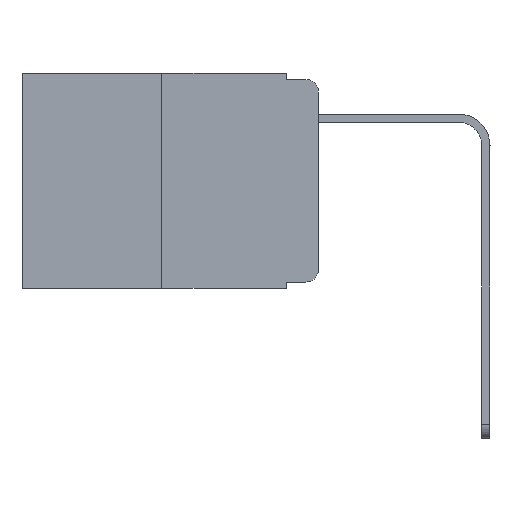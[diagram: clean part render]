
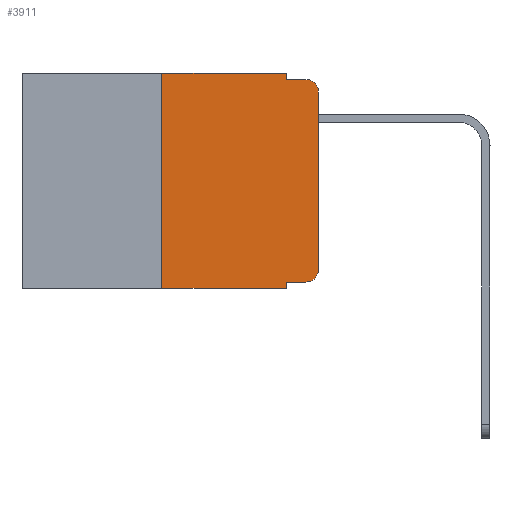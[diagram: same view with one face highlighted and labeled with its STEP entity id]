
A CAD part, left-side view. The second image highlights one B-rep face of the part: STEP entity #3911.
In plain terms, the highlighted planar face has unit normal (-1, 0, 0).
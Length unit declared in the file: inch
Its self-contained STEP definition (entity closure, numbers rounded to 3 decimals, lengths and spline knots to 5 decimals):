
#37 = DIRECTION ( 'NONE',  ( 0., -1., 0. ) ) ;
#202 = LINE ( 'NONE', #6691, #6022 ) ;
#251 = EDGE_CURVE ( 'NONE', #5769, #3876, #7273, .T. ) ;
#283 = DIRECTION ( 'NONE',  ( 0., 0., 1. ) ) ;
#401 = CARTESIAN_POINT ( 'NONE',  ( 0., 0.02, -0.03 ) ) ;
#458 = DIRECTION ( 'NONE',  ( -1., 0., 0. ) ) ;
#551 = CIRCLE ( 'NONE', #3579, 0.02 ) ;
#652 = EDGE_CURVE ( 'NONE', #7943, #8433, #551, .T. ) ;
#853 = VERTEX_POINT ( 'NONE', #8918 ) ;
#938 = CARTESIAN_POINT ( 'NONE',  ( 0., 0.473, -0.343 ) ) ;
#1070 = AXIS2_PLACEMENT_3D ( 'NONE', #401, #7732, #2834 ) ;
#1266 = EDGE_LOOP ( 'NONE', ( #7208, #2586, #8541, #6045, #2833, #6944, #1284, #6543, #9168, #8467 ) ) ;
#1284 = ORIENTED_EDGE ( 'NONE', *, *, #10166, .T. ) ;
#1497 = CARTESIAN_POINT ( 'NONE',  ( 0., 0., -0.313 ) ) ;
#1759 = VERTEX_POINT ( 'NONE', #6006 ) ;
#1990 = VERTEX_POINT ( 'NONE', #5425 ) ;
#2455 = EDGE_CURVE ( 'NONE', #1759, #5769, #9701, .T. ) ;
#2574 = DIRECTION ( 'NONE',  ( 0., -1., 0. ) ) ;
#2586 = ORIENTED_EDGE ( 'NONE', *, *, #9247, .T. ) ;
#2686 = CIRCLE ( 'NONE', #1070, 0.02 ) ;
#2694 = EDGE_CURVE ( 'NONE', #8433, #853, #202, .T. ) ;
#2833 = ORIENTED_EDGE ( 'NONE', *, *, #9095, .F. ) ;
#2834 = DIRECTION ( 'NONE',  ( 0., 0., -1. ) ) ;
#2859 = DIRECTION ( 'NONE',  ( 0., 0., -1. ) ) ;
#2900 = VERTEX_POINT ( 'NONE', #10089 ) ;
#3208 = LINE ( 'NONE', #4741, #5484 ) ;
#3267 = DIRECTION ( 'NONE',  ( 0., -1., 0. ) ) ;
#3305 = CARTESIAN_POINT ( 'NONE',  ( 0., 0.051, -0.01 ) ) ;
#3559 = CARTESIAN_POINT ( 'NONE',  ( 0., 0.25, 0. ) ) ;
#3579 = AXIS2_PLACEMENT_3D ( 'NONE', #3637, #458, #2859 ) ;
#3587 = CARTESIAN_POINT ( 'NONE',  ( 0., 0.25, 0. ) ) ;
#3637 = CARTESIAN_POINT ( 'NONE',  ( 0., 0.02, -0.313 ) ) ;
#3716 = DIRECTION ( 'NONE',  ( 0., 0., -1. ) ) ;
#3746 = PLANE ( 'NONE',  #9130 ) ;
#3876 = VERTEX_POINT ( 'NONE', #4237 ) ;
#3900 = CARTESIAN_POINT ( 'NONE',  ( 0., 0.051, 0. ) ) ;
#3911 = ADVANCED_FACE ( 'NONE', ( #8858 ), #3746, .F. ) ;
#4237 = CARTESIAN_POINT ( 'NONE',  ( 0., 0.02, -0.01 ) ) ;
#4452 = LINE ( 'NONE', #3559, #8730 ) ;
#4741 = CARTESIAN_POINT ( 'NONE',  ( 0., 0.473, 0. ) ) ;
#5026 = DIRECTION ( 'NONE',  ( 0., 0., 1. ) ) ;
#5117 = VECTOR ( 'NONE', #3267, 39.37008 ) ;
#5195 = VECTOR ( 'NONE', #9716, 39.37008 ) ;
#5201 = VERTEX_POINT ( 'NONE', #6834 ) ;
#5233 = VECTOR ( 'NONE', #6348, 39.37008 ) ;
#5425 = CARTESIAN_POINT ( 'NONE',  ( 0., 0.051, -0.343 ) ) ;
#5484 = VECTOR ( 'NONE', #5637, 39.37008 ) ;
#5637 = DIRECTION ( 'NONE',  ( 0., -1., 0. ) ) ;
#5722 = CARTESIAN_POINT ( 'NONE',  ( 0., 0.02, -0.333 ) ) ;
#5769 = VERTEX_POINT ( 'NONE', #8545 ) ;
#6006 = CARTESIAN_POINT ( 'NONE',  ( 0., 0.051, 0. ) ) ;
#6022 = VECTOR ( 'NONE', #5026, 39.37008 ) ;
#6045 = ORIENTED_EDGE ( 'NONE', *, *, #2455, .F. ) ;
#6348 = DIRECTION ( 'NONE',  ( 0., 0., -1. ) ) ;
#6463 = VECTOR ( 'NONE', #2574, 39.37008 ) ;
#6543 = ORIENTED_EDGE ( 'NONE', *, *, #8946, .F. ) ;
#6623 = CARTESIAN_POINT ( 'NONE',  ( 0., 0.051, 0. ) ) ;
#6691 = CARTESIAN_POINT ( 'NONE',  ( 0., 0., 0. ) ) ;
#6724 = LINE ( 'NONE', #7325, #6463 ) ;
#6834 = CARTESIAN_POINT ( 'NONE',  ( 0., 0.25, -0.343 ) ) ;
#6944 = ORIENTED_EDGE ( 'NONE', *, *, #8121, .F. ) ;
#7208 = ORIENTED_EDGE ( 'NONE', *, *, #2694, .T. ) ;
#7273 = LINE ( 'NONE', #3305, #5117 ) ;
#7325 = CARTESIAN_POINT ( 'NONE',  ( 0., 0.051, -0.333 ) ) ;
#7732 = DIRECTION ( 'NONE',  ( -1., 0., 0. ) ) ;
#7943 = VERTEX_POINT ( 'NONE', #5722 ) ;
#8121 = EDGE_CURVE ( 'NONE', #5201, #8650, #4452, .T. ) ;
#8275 = EDGE_CURVE ( 'NONE', #2900, #7943, #6724, .T. ) ;
#8433 = VERTEX_POINT ( 'NONE', #1497 ) ;
#8467 = ORIENTED_EDGE ( 'NONE', *, *, #652, .T. ) ;
#8541 = ORIENTED_EDGE ( 'NONE', *, *, #251, .F. ) ;
#8545 = CARTESIAN_POINT ( 'NONE',  ( 0., 0.051, -0.01 ) ) ;
#8650 = VERTEX_POINT ( 'NONE', #3587 ) ;
#8730 = VECTOR ( 'NONE', #283, 39.37008 ) ;
#8858 = FACE_OUTER_BOUND ( 'NONE', #1266, .T. ) ;
#8918 = CARTESIAN_POINT ( 'NONE',  ( 0., 0., -0.03 ) ) ;
#8946 = EDGE_CURVE ( 'NONE', #2900, #1990, #9876, .T. ) ;
#9095 = EDGE_CURVE ( 'NONE', #8650, #1759, #3208, .T. ) ;
#9130 = AXIS2_PLACEMENT_3D ( 'NONE', #9383, #9348, #3716 ) ;
#9168 = ORIENTED_EDGE ( 'NONE', *, *, #8275, .T. ) ;
#9247 = EDGE_CURVE ( 'NONE', #853, #3876, #2686, .T. ) ;
#9294 = LINE ( 'NONE', #938, #9417 ) ;
#9348 = DIRECTION ( 'NONE',  ( 1., 0., 0. ) ) ;
#9383 = CARTESIAN_POINT ( 'NONE',  ( 0., 0.473, 0. ) ) ;
#9417 = VECTOR ( 'NONE', #37, 39.37008 ) ;
#9701 = LINE ( 'NONE', #6623, #5195 ) ;
#9716 = DIRECTION ( 'NONE',  ( 0., 0., -1. ) ) ;
#9876 = LINE ( 'NONE', #3900, #5233 ) ;
#10089 = CARTESIAN_POINT ( 'NONE',  ( 0., 0.051, -0.333 ) ) ;
#10166 = EDGE_CURVE ( 'NONE', #5201, #1990, #9294, .T. ) ;
